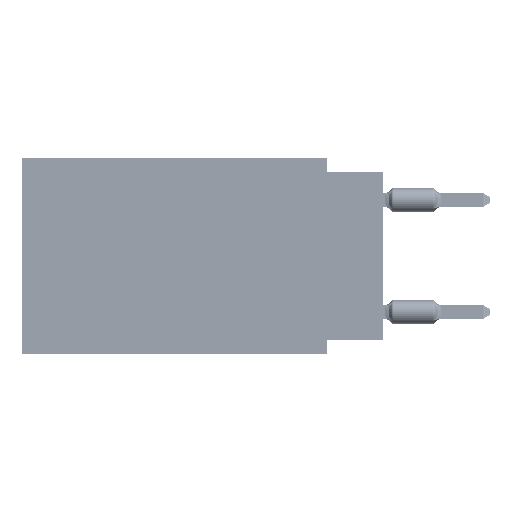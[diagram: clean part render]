
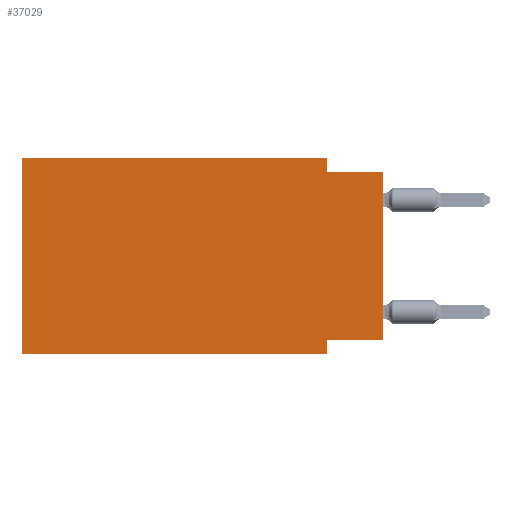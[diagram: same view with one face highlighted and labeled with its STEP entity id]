
A CAD part, left-side view. The second image highlights one B-rep face of the part: STEP entity #37029.
In plain terms, the highlighted planar face has unit normal (-1, 0, 0).
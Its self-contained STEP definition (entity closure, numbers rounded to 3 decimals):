
#1229 = DIRECTION ( 'NONE',  ( 0., 0., -1. ) ) ;
#2024 = CARTESIAN_POINT ( 'NONE',  ( 0., 2.54, 0. ) ) ;
#2117 = ORIENTED_EDGE ( 'NONE', *, *, #35391, .T. ) ;
#3179 = ORIENTED_EDGE ( 'NONE', *, *, #32027, .F. ) ;
#3952 = CARTESIAN_POINT ( 'NONE',  ( 0., 0., -0.635 ) ) ;
#4783 = LINE ( 'NONE', #3952, #26613 ) ;
#6193 = DIRECTION ( 'NONE',  ( 0., 0., -1. ) ) ;
#7151 = CARTESIAN_POINT ( 'NONE',  ( 0., 16.383, 0. ) ) ;
#11199 = VERTEX_POINT ( 'NONE', #35995 ) ;
#12143 = VECTOR ( 'NONE', #28650, 1000. ) ;
#15844 = CARTESIAN_POINT ( 'NONE',  ( 0., 16.383, -8.89 ) ) ;
#16521 = CARTESIAN_POINT ( 'NONE',  ( 0., 2.54, -8.89 ) ) ;
#16771 = ORIENTED_EDGE ( 'NONE', *, *, #73682, .F. ) ;
#18964 = DIRECTION ( 'NONE',  ( 1., 0., 0. ) ) ;
#19465 = DIRECTION ( 'NONE',  ( 0., 0., 1. ) ) ;
#20271 = VERTEX_POINT ( 'NONE', #29987 ) ;
#20467 = CARTESIAN_POINT ( 'NONE',  ( 0., 0., -0.635 ) ) ;
#20699 = EDGE_CURVE ( 'NONE', #24969, #76838, #61557, .T. ) ;
#21454 = VECTOR ( 'NONE', #35908, 1000. ) ;
#22120 = ORIENTED_EDGE ( 'NONE', *, *, #26954, .F. ) ;
#23148 = CARTESIAN_POINT ( 'NONE',  ( 0., 16.383, 0. ) ) ;
#24232 = ORIENTED_EDGE ( 'NONE', *, *, #76940, .F. ) ;
#24969 = VERTEX_POINT ( 'NONE', #48610 ) ;
#26613 = VECTOR ( 'NONE', #55420, 1000. ) ;
#26954 = EDGE_CURVE ( 'NONE', #76838, #66989, #49666, .T. ) ;
#28650 = DIRECTION ( 'NONE',  ( 0., -1., 0. ) ) ;
#29804 = DIRECTION ( 'NONE',  ( 0., 0., 1. ) ) ;
#29987 = CARTESIAN_POINT ( 'NONE',  ( 0., 16.383, -8.89 ) ) ;
#30218 = LINE ( 'NONE', #55978, #76351 ) ;
#30832 = CARTESIAN_POINT ( 'NONE',  ( 0., 0., -8.255 ) ) ;
#32027 = EDGE_CURVE ( 'NONE', #66989, #50310, #4783, .T. ) ;
#33354 = CARTESIAN_POINT ( 'NONE',  ( 0., 0., 0. ) ) ;
#33982 = AXIS2_PLACEMENT_3D ( 'NONE', #7151, #18964, #1229 ) ;
#35391 = EDGE_CURVE ( 'NONE', #55882, #50310, #45213, .T. ) ;
#35908 = DIRECTION ( 'NONE',  ( 0., 0., -1. ) ) ;
#35995 = CARTESIAN_POINT ( 'NONE',  ( 0., 2.54, -8.255 ) ) ;
#37029 = ADVANCED_FACE ( 'NONE', ( #58200 ), #52698, .F. ) ;
#41711 = EDGE_CURVE ( 'NONE', #20271, #60888, #53826, .T. ) ;
#43082 = DIRECTION ( 'NONE',  ( 0., 1., 0. ) ) ;
#45213 = LINE ( 'NONE', #33354, #71455 ) ;
#46247 = DIRECTION ( 'NONE',  ( 0., -1., 0. ) ) ;
#48610 = CARTESIAN_POINT ( 'NONE',  ( 0., 16.383, 0. ) ) ;
#49666 = LINE ( 'NONE', #75815, #51830 ) ;
#50250 = LINE ( 'NONE', #30832, #71701 ) ;
#50310 = VERTEX_POINT ( 'NONE', #20467 ) ;
#51830 = VECTOR ( 'NONE', #6193, 1000. ) ;
#52698 = PLANE ( 'NONE',  #33982 ) ;
#53181 = EDGE_CURVE ( 'NONE', #55882, #11199, #50250, .T. ) ;
#53593 = ORIENTED_EDGE ( 'NONE', *, *, #41711, .T. ) ;
#53826 = LINE ( 'NONE', #15844, #66693 ) ;
#54693 = CARTESIAN_POINT ( 'NONE',  ( 0., 2.54, -8.89 ) ) ;
#55420 = DIRECTION ( 'NONE',  ( 0., -1., 0. ) ) ;
#55882 = VERTEX_POINT ( 'NONE', #68085 ) ;
#55978 = CARTESIAN_POINT ( 'NONE',  ( 0., 16.383, 0. ) ) ;
#57038 = CARTESIAN_POINT ( 'NONE',  ( 0., 2.54, -0.635 ) ) ;
#58200 = FACE_OUTER_BOUND ( 'NONE', #61827, .T. ) ;
#60888 = VERTEX_POINT ( 'NONE', #54693 ) ;
#61557 = LINE ( 'NONE', #23148, #12143 ) ;
#61827 = EDGE_LOOP ( 'NONE', ( #2117, #3179, #22120, #77043, #24232, #53593, #16771, #72882 ) ) ;
#66693 = VECTOR ( 'NONE', #46247, 1000. ) ;
#66989 = VERTEX_POINT ( 'NONE', #57038 ) ;
#68085 = CARTESIAN_POINT ( 'NONE',  ( 0., 0., -8.255 ) ) ;
#71455 = VECTOR ( 'NONE', #19465, 1000. ) ;
#71701 = VECTOR ( 'NONE', #43082, 1000. ) ;
#72882 = ORIENTED_EDGE ( 'NONE', *, *, #53181, .F. ) ;
#73682 = EDGE_CURVE ( 'NONE', #11199, #60888, #74719, .T. ) ;
#74719 = LINE ( 'NONE', #16521, #21454 ) ;
#75815 = CARTESIAN_POINT ( 'NONE',  ( 0., 2.54, 0. ) ) ;
#76351 = VECTOR ( 'NONE', #29804, 1000. ) ;
#76838 = VERTEX_POINT ( 'NONE', #2024 ) ;
#76940 = EDGE_CURVE ( 'NONE', #20271, #24969, #30218, .T. ) ;
#77043 = ORIENTED_EDGE ( 'NONE', *, *, #20699, .F. ) ;
